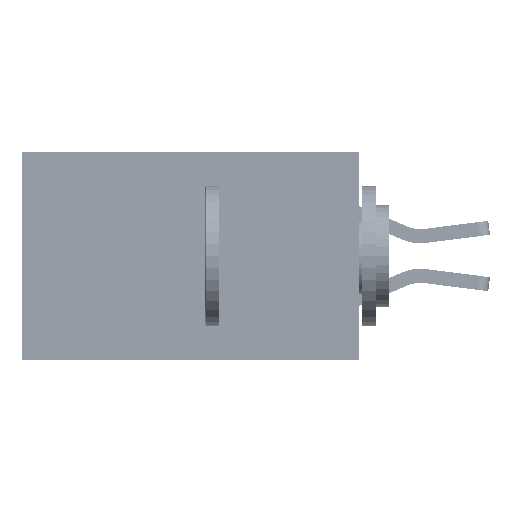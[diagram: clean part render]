
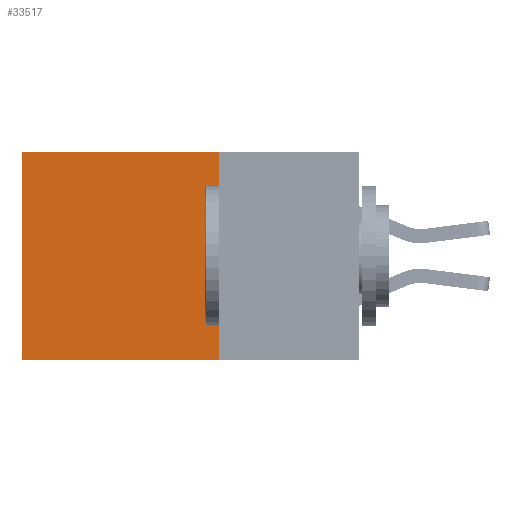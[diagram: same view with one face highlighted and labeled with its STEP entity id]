
A CAD part, left-side view. The second image highlights one B-rep face of the part: STEP entity #33517.
In plain terms, the highlighted planar face has unit normal (-1, 0, 0).
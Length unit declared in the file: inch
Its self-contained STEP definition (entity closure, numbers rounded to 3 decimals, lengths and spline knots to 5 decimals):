
#1464 = LINE ( 'NONE', #8451, #20933 ) ;
#2354 = LINE ( 'NONE', #26706, #21804 ) ;
#2629 = CARTESIAN_POINT ( 'NONE',  ( 0.2875, 0.6, 0. ) ) ;
#3630 = EDGE_LOOP ( 'NONE', ( #20507, #26434, #28828, #7607 ) ) ;
#4918 = DIRECTION ( 'NONE',  ( 0., 1., 0. ) ) ;
#6367 = VERTEX_POINT ( 'NONE', #39917 ) ;
#7039 = VECTOR ( 'NONE', #41281, 39.37008 ) ;
#7607 = ORIENTED_EDGE ( 'NONE', *, *, #14825, .T. ) ;
#7812 = CARTESIAN_POINT ( 'NONE',  ( 0.2875, 0.25, -0.37 ) ) ;
#8451 = CARTESIAN_POINT ( 'NONE',  ( 0.2875, 0.25, 0. ) ) ;
#8623 = EDGE_CURVE ( 'NONE', #6367, #11472, #36698, .T. ) ;
#9340 = CARTESIAN_POINT ( 'NONE',  ( 0.2875, 0.6, -0.37 ) ) ;
#10152 = CARTESIAN_POINT ( 'NONE',  ( 0.2875, 0.25, -0.37 ) ) ;
#11472 = VERTEX_POINT ( 'NONE', #9340 ) ;
#12374 = EDGE_CURVE ( 'NONE', #44559, #36321, #2354, .T. ) ;
#14158 = EDGE_CURVE ( 'NONE', #36321, #11472, #50040, .T. ) ;
#14825 = EDGE_CURVE ( 'NONE', #44559, #6367, #1464, .T. ) ;
#16412 = PLANE ( 'NONE',  #19150 ) ;
#19150 = AXIS2_PLACEMENT_3D ( 'NONE', #43502, #47397, #24215 ) ;
#20507 = ORIENTED_EDGE ( 'NONE', *, *, #8623, .T. ) ;
#20933 = VECTOR ( 'NONE', #43296, 39.37008 ) ;
#21804 = VECTOR ( 'NONE', #30597, 39.37008 ) ;
#24215 = DIRECTION ( 'NONE',  ( 0., 0., -1. ) ) ;
#26434 = ORIENTED_EDGE ( 'NONE', *, *, #14158, .F. ) ;
#26706 = CARTESIAN_POINT ( 'NONE',  ( 0.2875, 0.25, 0. ) ) ;
#28828 = ORIENTED_EDGE ( 'NONE', *, *, #12374, .F. ) ;
#30597 = DIRECTION ( 'NONE',  ( 0., 0., -1. ) ) ;
#33517 = ADVANCED_FACE ( 'NONE', ( #37852 ), #16412, .F. ) ;
#36321 = VERTEX_POINT ( 'NONE', #7812 ) ;
#36698 = LINE ( 'NONE', #2629, #7039 ) ;
#37852 = FACE_OUTER_BOUND ( 'NONE', #3630, .T. ) ;
#39768 = VECTOR ( 'NONE', #4918, 39.37008 ) ;
#39917 = CARTESIAN_POINT ( 'NONE',  ( 0.2875, 0.6, 0. ) ) ;
#40233 = CARTESIAN_POINT ( 'NONE',  ( 0.2875, 0.25, 0. ) ) ;
#41281 = DIRECTION ( 'NONE',  ( 0., 0., -1. ) ) ;
#43296 = DIRECTION ( 'NONE',  ( 0., 1., 0. ) ) ;
#43502 = CARTESIAN_POINT ( 'NONE',  ( 0.2875, 0.25, 0. ) ) ;
#44559 = VERTEX_POINT ( 'NONE', #40233 ) ;
#47397 = DIRECTION ( 'NONE',  ( 1., 0., 0. ) ) ;
#50040 = LINE ( 'NONE', #10152, #39768 ) ;
